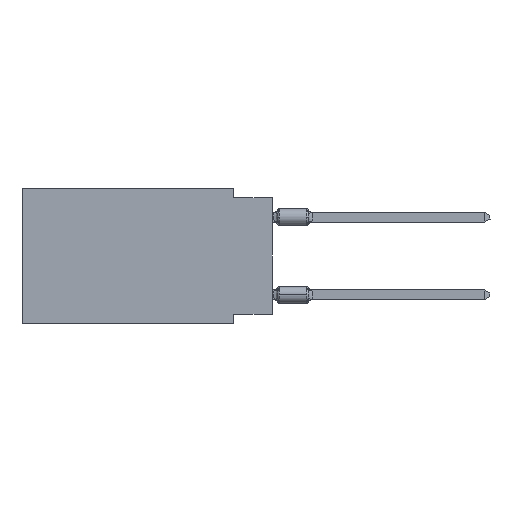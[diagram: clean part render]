
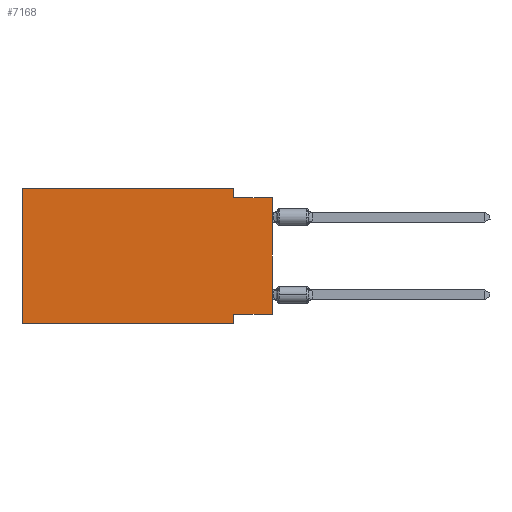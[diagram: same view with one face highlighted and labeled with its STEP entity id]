
A CAD part, left-side view. The second image highlights one B-rep face of the part: STEP entity #7168.
In plain terms, the highlighted planar face has unit normal (-1, 0, 0).
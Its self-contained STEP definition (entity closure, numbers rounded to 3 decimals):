
#98 = EDGE_CURVE ( 'NONE', #26827, #545, #8625, .T. ) ;
#213 = LINE ( 'NONE', #12927, #19896 ) ;
#545 = VERTEX_POINT ( 'NONE', #12598 ) ;
#1095 = DIRECTION ( 'NONE',  ( 0., 0., 1. ) ) ;
#1454 = VECTOR ( 'NONE', #9202, 1000. ) ;
#1723 = CARTESIAN_POINT ( 'NONE',  ( 0., 16.383, 0. ) ) ;
#1858 = FACE_OUTER_BOUND ( 'NONE', #12655, .T. ) ;
#2304 = DIRECTION ( 'NONE',  ( 0., -1., 0. ) ) ;
#2671 = EDGE_CURVE ( 'NONE', #4602, #25150, #25574, .T. ) ;
#2737 = VECTOR ( 'NONE', #1095, 1000. ) ;
#3598 = CARTESIAN_POINT ( 'NONE',  ( 0., 16.383, 0. ) ) ;
#4585 = CARTESIAN_POINT ( 'NONE',  ( 0., 16.383, -8.89 ) ) ;
#4602 = VERTEX_POINT ( 'NONE', #9843 ) ;
#5168 = ORIENTED_EDGE ( 'NONE', *, *, #26750, .F. ) ;
#5177 = CARTESIAN_POINT ( 'NONE',  ( 0., 0., -0.635 ) ) ;
#5804 = ORIENTED_EDGE ( 'NONE', *, *, #5907, .F. ) ;
#5855 = DIRECTION ( 'NONE',  ( 1., 0., 0. ) ) ;
#5907 = EDGE_CURVE ( 'NONE', #25640, #12528, #8166, .T. ) ;
#6019 = DIRECTION ( 'NONE',  ( 0., -1., 0. ) ) ;
#6187 = VERTEX_POINT ( 'NONE', #19524 ) ;
#6714 = LINE ( 'NONE', #10861, #1454 ) ;
#7024 = CARTESIAN_POINT ( 'NONE',  ( 0., 2.54, -8.255 ) ) ;
#7168 = ADVANCED_FACE ( 'NONE', ( #1858 ), #22890, .F. ) ;
#8166 = LINE ( 'NONE', #19108, #24194 ) ;
#8502 = DIRECTION ( 'NONE',  ( 0., -1., 0. ) ) ;
#8620 = DIRECTION ( 'NONE',  ( 0., 0., -1. ) ) ;
#8625 = LINE ( 'NONE', #18633, #26481 ) ;
#8634 = VERTEX_POINT ( 'NONE', #4585 ) ;
#8853 = ORIENTED_EDGE ( 'NONE', *, *, #17762, .F. ) ;
#8936 = ORIENTED_EDGE ( 'NONE', *, *, #21386, .F. ) ;
#9114 = ORIENTED_EDGE ( 'NONE', *, *, #27060, .T. ) ;
#9202 = DIRECTION ( 'NONE',  ( 0., 0., 1. ) ) ;
#9843 = CARTESIAN_POINT ( 'NONE',  ( 0., 2.54, -0.635 ) ) ;
#10174 = CARTESIAN_POINT ( 'NONE',  ( 0., 0., -0.635 ) ) ;
#10260 = DIRECTION ( 'NONE',  ( 0., 0., -1. ) ) ;
#10424 = ORIENTED_EDGE ( 'NONE', *, *, #21730, .T. ) ;
#10861 = CARTESIAN_POINT ( 'NONE',  ( 0., 0., 0. ) ) ;
#12528 = VERTEX_POINT ( 'NONE', #7024 ) ;
#12598 = CARTESIAN_POINT ( 'NONE',  ( 0., 2.54, 0. ) ) ;
#12655 = EDGE_LOOP ( 'NONE', ( #10424, #24085, #8853, #16691, #8936, #9114, #5168, #5804 ) ) ;
#12927 = CARTESIAN_POINT ( 'NONE',  ( 0., 2.54, 0. ) ) ;
#13975 = CARTESIAN_POINT ( 'NONE',  ( 0., 0., -8.255 ) ) ;
#14332 = VECTOR ( 'NONE', #6019, 1000. ) ;
#16691 = ORIENTED_EDGE ( 'NONE', *, *, #98, .F. ) ;
#17271 = CARTESIAN_POINT ( 'NONE',  ( 0., 2.54, -8.89 ) ) ;
#17762 = EDGE_CURVE ( 'NONE', #545, #4602, #213, .T. ) ;
#18633 = CARTESIAN_POINT ( 'NONE',  ( 0., 16.383, 0. ) ) ;
#18641 = CARTESIAN_POINT ( 'NONE',  ( 0., 16.383, -8.89 ) ) ;
#19108 = CARTESIAN_POINT ( 'NONE',  ( 0., 0., -8.255 ) ) ;
#19524 = CARTESIAN_POINT ( 'NONE',  ( 0., 2.54, -8.89 ) ) ;
#19768 = AXIS2_PLACEMENT_3D ( 'NONE', #1723, #5855, #10260 ) ;
#19896 = VECTOR ( 'NONE', #8620, 1000. ) ;
#20042 = LINE ( 'NONE', #3598, #2737 ) ;
#21190 = DIRECTION ( 'NONE',  ( 0., 1., 0. ) ) ;
#21386 = EDGE_CURVE ( 'NONE', #8634, #26827, #20042, .T. ) ;
#21415 = CARTESIAN_POINT ( 'NONE',  ( 0., 16.383, 0. ) ) ;
#21730 = EDGE_CURVE ( 'NONE', #25640, #25150, #6714, .T. ) ;
#21830 = DIRECTION ( 'NONE',  ( 0., 0., -1. ) ) ;
#22890 = PLANE ( 'NONE',  #19768 ) ;
#23655 = LINE ( 'NONE', #17271, #24376 ) ;
#24085 = ORIENTED_EDGE ( 'NONE', *, *, #2671, .F. ) ;
#24194 = VECTOR ( 'NONE', #21190, 1000. ) ;
#24376 = VECTOR ( 'NONE', #21830, 1000. ) ;
#24704 = VECTOR ( 'NONE', #8502, 1000. ) ;
#25150 = VERTEX_POINT ( 'NONE', #5177 ) ;
#25186 = LINE ( 'NONE', #18641, #24704 ) ;
#25574 = LINE ( 'NONE', #10174, #14332 ) ;
#25640 = VERTEX_POINT ( 'NONE', #13975 ) ;
#26481 = VECTOR ( 'NONE', #2304, 1000. ) ;
#26750 = EDGE_CURVE ( 'NONE', #12528, #6187, #23655, .T. ) ;
#26827 = VERTEX_POINT ( 'NONE', #21415 ) ;
#27060 = EDGE_CURVE ( 'NONE', #8634, #6187, #25186, .T. ) ;
